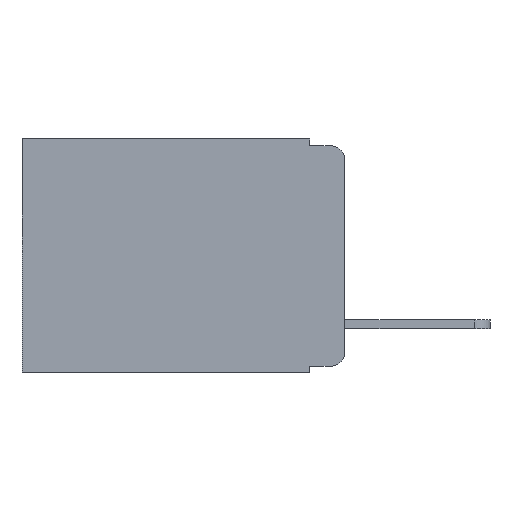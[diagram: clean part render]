
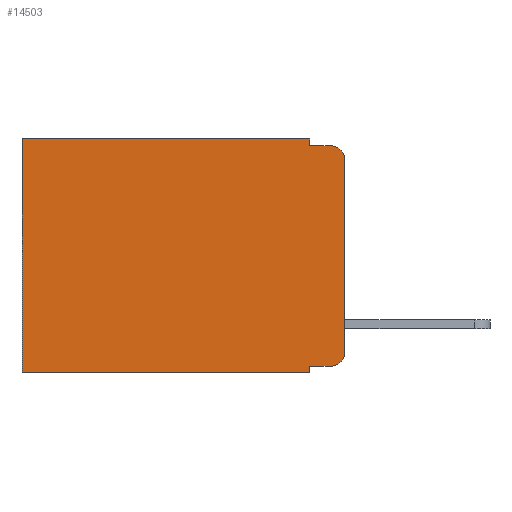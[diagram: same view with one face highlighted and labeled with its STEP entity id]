
A CAD part, left-side view. The second image highlights one B-rep face of the part: STEP entity #14503.
In plain terms, the highlighted planar face has unit normal (-1, 0, 0).
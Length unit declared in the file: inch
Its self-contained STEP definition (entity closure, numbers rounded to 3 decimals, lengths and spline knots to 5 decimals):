
#203 = DIRECTION ( 'NONE',  ( 0., 1., 0. ) ) ;
#267 = LINE ( 'NONE', #5021, #13559 ) ;
#439 = ORIENTED_EDGE ( 'NONE', *, *, #14111, .T. ) ;
#465 = VERTEX_POINT ( 'NONE', #4095 ) ;
#606 = VERTEX_POINT ( 'NONE', #15710 ) ;
#625 = AXIS2_PLACEMENT_3D ( 'NONE', #11328, #3422, #12676 ) ;
#1153 = FACE_OUTER_BOUND ( 'NONE', #17099, .T. ) ;
#1162 = VERTEX_POINT ( 'NONE', #2169 ) ;
#1577 = ORIENTED_EDGE ( 'NONE', *, *, #2242, .F. ) ;
#1747 = ORIENTED_EDGE ( 'NONE', *, *, #15059, .T. ) ;
#2072 = CARTESIAN_POINT ( 'NONE',  ( 0.298, 0., 0. ) ) ;
#2079 = LINE ( 'NONE', #13792, #12223 ) ;
#2169 = CARTESIAN_POINT ( 'NONE',  ( 0.298, 0.02, -0.333 ) ) ;
#2242 = EDGE_CURVE ( 'NONE', #10873, #2474, #267, .T. ) ;
#2474 = VERTEX_POINT ( 'NONE', #5157 ) ;
#2666 = ORIENTED_EDGE ( 'NONE', *, *, #3057, .F. ) ;
#3057 = EDGE_CURVE ( 'NONE', #465, #14371, #2079, .T. ) ;
#3134 = EDGE_CURVE ( 'NONE', #13460, #10873, #10989, .T. ) ;
#3351 = DIRECTION ( 'NONE',  ( 0., -1., 0. ) ) ;
#3422 = DIRECTION ( 'NONE',  ( -1., 0., 0. ) ) ;
#3642 = CIRCLE ( 'NONE', #625, 0.02 ) ;
#3665 = DIRECTION ( 'NONE',  ( 0., 0., -1. ) ) ;
#3981 = EDGE_CURVE ( 'NONE', #12134, #1162, #12426, .T. ) ;
#4095 = CARTESIAN_POINT ( 'NONE',  ( 0.298, 0.051, -0.343 ) ) ;
#4183 = PLANE ( 'NONE',  #4544 ) ;
#4263 = CARTESIAN_POINT ( 'NONE',  ( 0.298, 0.051, -0.333 ) ) ;
#4523 = DIRECTION ( 'NONE',  ( -1., 0., 0. ) ) ;
#4544 = AXIS2_PLACEMENT_3D ( 'NONE', #14752, #6847, #16042 ) ;
#4680 = CARTESIAN_POINT ( 'NONE',  ( 0.298, 0.051, -0.333 ) ) ;
#5021 = CARTESIAN_POINT ( 'NONE',  ( 0.298, 0.051, -0.01 ) ) ;
#5029 = DIRECTION ( 'NONE',  ( 0., -1., 0. ) ) ;
#5157 = CARTESIAN_POINT ( 'NONE',  ( 0.298, 0.02, -0.01 ) ) ;
#5682 = LINE ( 'NONE', #2072, #15780 ) ;
#5759 = CARTESIAN_POINT ( 'NONE',  ( 0.298, 0.051, 0. ) ) ;
#6153 = ORIENTED_EDGE ( 'NONE', *, *, #14700, .T. ) ;
#6243 = VECTOR ( 'NONE', #7336, 39.37008 ) ;
#6847 = DIRECTION ( 'NONE',  ( 1., 0., 0. ) ) ;
#6862 = CARTESIAN_POINT ( 'NONE',  ( 0.298, 0., 0. ) ) ;
#7282 = DIRECTION ( 'NONE',  ( 0., 0., -1. ) ) ;
#7336 = DIRECTION ( 'NONE',  ( 0., 0., -1. ) ) ;
#7431 = ORIENTED_EDGE ( 'NONE', *, *, #3134, .F. ) ;
#7442 = CARTESIAN_POINT ( 'NONE',  ( 0.298, 0.051, -0.01 ) ) ;
#7535 = CARTESIAN_POINT ( 'NONE',  ( 0.298, 0.051, 0. ) ) ;
#7891 = CARTESIAN_POINT ( 'NONE',  ( 0.298, 0.473, 0. ) ) ;
#8443 = ORIENTED_EDGE ( 'NONE', *, *, #15883, .F. ) ;
#9108 = ORIENTED_EDGE ( 'NONE', *, *, #10827, .T. ) ;
#9254 = CIRCLE ( 'NONE', #9402, 0.02 ) ;
#9344 = VECTOR ( 'NONE', #3351, 39.37008 ) ;
#9379 = VECTOR ( 'NONE', #7282, 39.37008 ) ;
#9402 = AXIS2_PLACEMENT_3D ( 'NONE', #12430, #4523, #13773 ) ;
#9418 = ORIENTED_EDGE ( 'NONE', *, *, #15304, .F. ) ;
#9776 = DIRECTION ( 'NONE',  ( 0., 1., 0. ) ) ;
#10827 = EDGE_CURVE ( 'NONE', #11979, #14371, #13708, .T. ) ;
#10873 = VERTEX_POINT ( 'NONE', #7442 ) ;
#10989 = LINE ( 'NONE', #7535, #14918 ) ;
#11328 = CARTESIAN_POINT ( 'NONE',  ( 0.298, 0.02, -0.313 ) ) ;
#11849 = CARTESIAN_POINT ( 'NONE',  ( 0.298, 0.473, -0.343 ) ) ;
#11979 = VERTEX_POINT ( 'NONE', #7891 ) ;
#12134 = VERTEX_POINT ( 'NONE', #4263 ) ;
#12223 = VECTOR ( 'NONE', #9776, 39.37008 ) ;
#12426 = LINE ( 'NONE', #4680, #9344 ) ;
#12430 = CARTESIAN_POINT ( 'NONE',  ( 0.298, 0.02, -0.03 ) ) ;
#12654 = DIRECTION ( 'NONE',  ( 0., 0., -1. ) ) ;
#12676 = DIRECTION ( 'NONE',  ( 0., 0., -1. ) ) ;
#12877 = LINE ( 'NONE', #16455, #9379 ) ;
#12911 = VECTOR ( 'NONE', #203, 39.37008 ) ;
#13460 = VERTEX_POINT ( 'NONE', #5759 ) ;
#13559 = VECTOR ( 'NONE', #5029, 39.37008 ) ;
#13708 = LINE ( 'NONE', #16508, #6243 ) ;
#13757 = LINE ( 'NONE', #6862, #12911 ) ;
#13773 = DIRECTION ( 'NONE',  ( 0., 0., -1. ) ) ;
#13792 = CARTESIAN_POINT ( 'NONE',  ( 0.298, 0., -0.343 ) ) ;
#14110 = VERTEX_POINT ( 'NONE', #16267 ) ;
#14111 = EDGE_CURVE ( 'NONE', #14110, #2474, #9254, .T. ) ;
#14371 = VERTEX_POINT ( 'NONE', #11849 ) ;
#14503 = ADVANCED_FACE ( 'NONE', ( #1153 ), #4183, .F. ) ;
#14700 = EDGE_CURVE ( 'NONE', #1162, #606, #3642, .T. ) ;
#14752 = CARTESIAN_POINT ( 'NONE',  ( 0.298, 0., 0. ) ) ;
#14918 = VECTOR ( 'NONE', #3665, 39.37008 ) ;
#15059 = EDGE_CURVE ( 'NONE', #13460, #11979, #13757, .T. ) ;
#15304 = EDGE_CURVE ( 'NONE', #14110, #606, #5682, .T. ) ;
#15710 = CARTESIAN_POINT ( 'NONE',  ( 0.298, 0., -0.313 ) ) ;
#15780 = VECTOR ( 'NONE', #12654, 39.37008 ) ;
#15883 = EDGE_CURVE ( 'NONE', #12134, #465, #12877, .T. ) ;
#16042 = DIRECTION ( 'NONE',  ( 0., 0., -1. ) ) ;
#16267 = CARTESIAN_POINT ( 'NONE',  ( 0.298, 0., -0.03 ) ) ;
#16455 = CARTESIAN_POINT ( 'NONE',  ( 0.298, 0.051, 0. ) ) ;
#16508 = CARTESIAN_POINT ( 'NONE',  ( 0.298, 0.473, 0. ) ) ;
#16530 = ORIENTED_EDGE ( 'NONE', *, *, #3981, .T. ) ;
#17099 = EDGE_LOOP ( 'NONE', ( #9418, #439, #1577, #7431, #1747, #9108, #2666, #8443, #16530, #6153 ) ) ;
